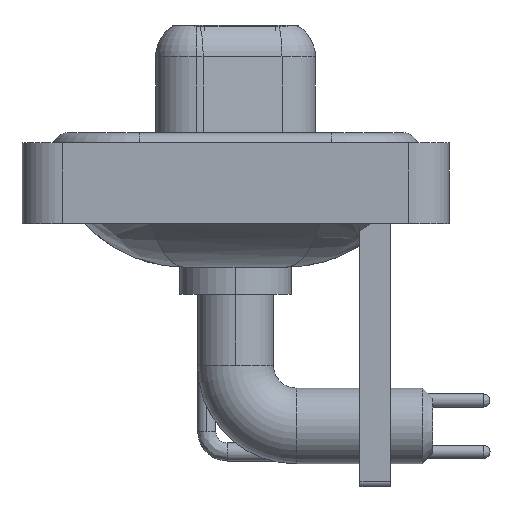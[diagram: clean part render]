
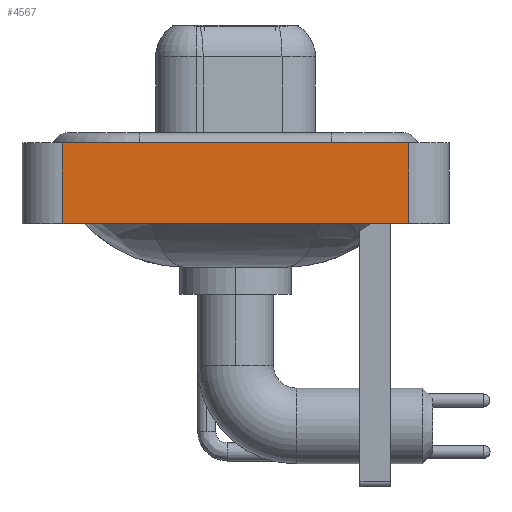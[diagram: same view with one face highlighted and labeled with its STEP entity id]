
A CAD part, left-side view. The second image highlights one B-rep face of the part: STEP entity #4567.
In plain terms, the highlighted planar face has unit normal (-1, 0, 0).
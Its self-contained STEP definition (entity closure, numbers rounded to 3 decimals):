
#1136 = DIRECTION ( 'NONE',  ( 0., 0., 1. ) ) ;
#1641 = DIRECTION ( 'NONE',  ( 0., 0., 1. ) ) ;
#2141 = EDGE_CURVE ( 'NONE', #3656, #13972, #15824, .T. ) ;
#3013 = ORIENTED_EDGE ( 'NONE', *, *, #10899, .T. ) ;
#3656 = VERTEX_POINT ( 'NONE', #12044 ) ;
#3837 = AXIS2_PLACEMENT_3D ( 'NONE', #19343, #15644, #1136 ) ;
#4224 = EDGE_CURVE ( 'NONE', #15949, #4704, #15898, .T. ) ;
#4567 = ADVANCED_FACE ( 'NONE', ( #20538 ), #18737, .T. ) ;
#4704 = VERTEX_POINT ( 'NONE', #17318 ) ;
#4931 = CARTESIAN_POINT ( 'NONE',  ( -7.35, 8.55, -3.6 ) ) ;
#5588 = CARTESIAN_POINT ( 'NONE',  ( -7.35, -8.55, 0.4 ) ) ;
#5821 = LINE ( 'NONE', #5588, #18655 ) ;
#6600 = VECTOR ( 'NONE', #15175, 1000. ) ;
#6724 = DIRECTION ( 'NONE',  ( 0., 0., 1. ) ) ;
#6804 = CARTESIAN_POINT ( 'NONE',  ( -7.35, -8.55, -3.6 ) ) ;
#8019 = VECTOR ( 'NONE', #1641, 1000. ) ;
#8530 = CARTESIAN_POINT ( 'NONE',  ( -7.35, 8.55, 0.4 ) ) ;
#10885 = ORIENTED_EDGE ( 'NONE', *, *, #14569, .F. ) ;
#10899 = EDGE_CURVE ( 'NONE', #3656, #15949, #16975, .T. ) ;
#11769 = VECTOR ( 'NONE', #6724, 1000. ) ;
#12044 = CARTESIAN_POINT ( 'NONE',  ( -7.35, 8.55, -3.6 ) ) ;
#12890 = EDGE_LOOP ( 'NONE', ( #23345, #10885, #16953, #3013 ) ) ;
#13121 = DIRECTION ( 'NONE',  ( 0., -1., 0. ) ) ;
#13972 = VERTEX_POINT ( 'NONE', #8530 ) ;
#14569 = EDGE_CURVE ( 'NONE', #13972, #4704, #5821, .T. ) ;
#15175 = DIRECTION ( 'NONE',  ( 0., -1., 0. ) ) ;
#15644 = DIRECTION ( 'NONE',  ( -1., 0., 0. ) ) ;
#15824 = LINE ( 'NONE', #4931, #11769 ) ;
#15898 = LINE ( 'NONE', #6804, #8019 ) ;
#15949 = VERTEX_POINT ( 'NONE', #21781 ) ;
#16953 = ORIENTED_EDGE ( 'NONE', *, *, #2141, .F. ) ;
#16975 = LINE ( 'NONE', #20561, #6600 ) ;
#17318 = CARTESIAN_POINT ( 'NONE',  ( -7.35, -8.55, 0.4 ) ) ;
#18655 = VECTOR ( 'NONE', #13121, 1000. ) ;
#18737 = PLANE ( 'NONE',  #3837 ) ;
#19343 = CARTESIAN_POINT ( 'NONE',  ( -7.35, -8.55, -3.6 ) ) ;
#20538 = FACE_OUTER_BOUND ( 'NONE', #12890, .T. ) ;
#20561 = CARTESIAN_POINT ( 'NONE',  ( -7.35, -8.55, -3.6 ) ) ;
#21781 = CARTESIAN_POINT ( 'NONE',  ( -7.35, -8.55, -3.6 ) ) ;
#23345 = ORIENTED_EDGE ( 'NONE', *, *, #4224, .T. ) ;
